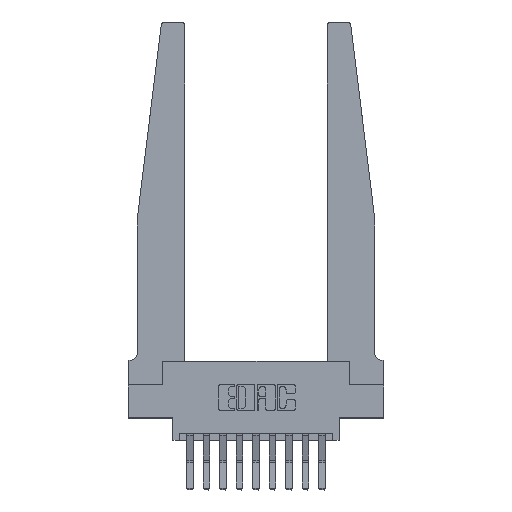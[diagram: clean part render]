
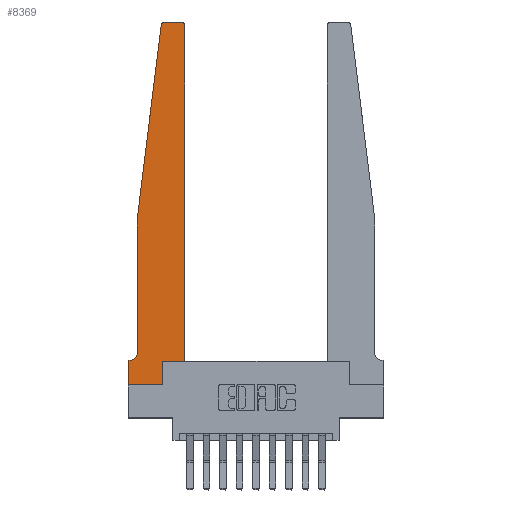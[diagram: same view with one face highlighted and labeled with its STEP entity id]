
A CAD part, top view. The second image highlights one B-rep face of the part: STEP entity #8369.
In plain terms, the highlighted planar face has unit normal (0, 0, 1).
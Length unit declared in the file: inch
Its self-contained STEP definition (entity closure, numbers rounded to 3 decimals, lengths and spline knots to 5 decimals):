
#51 = ORIENTED_EDGE ( 'NONE', *, *, #7504, .T. ) ;
#128 = CARTESIAN_POINT ( 'NONE',  ( 0.425, 0.18, 0.37 ) ) ;
#229 = AXIS2_PLACEMENT_3D ( 'NONE', #2099, #6623, #13943 ) ;
#252 = AXIS2_PLACEMENT_3D ( 'NONE', #6421, #1732, #11304 ) ;
#266 = CARTESIAN_POINT ( 'NONE',  ( 0.065, 1.25, 0.37 ) ) ;
#479 = LINE ( 'NONE', #1680, #1055 ) ;
#628 = AXIS2_PLACEMENT_3D ( 'NONE', #4813, #907, #8316 ) ;
#907 = DIRECTION ( 'NONE',  ( 0., 0., -1. ) ) ;
#963 = ORIENTED_EDGE ( 'NONE', *, *, #7296, .T. ) ;
#1006 = VECTOR ( 'NONE', #1713, 39.37008 ) ;
#1055 = VECTOR ( 'NONE', #5318, 39.37008 ) ;
#1065 = DIRECTION ( 'NONE',  ( -0.122, -0.992, 0. ) ) ;
#1325 = CARTESIAN_POINT ( 'NONE',  ( 0.2605, 0., 0.37 ) ) ;
#1422 = EDGE_CURVE ( 'NONE', #2027, #12959, #5453, .T. ) ;
#1680 = CARTESIAN_POINT ( 'NONE',  ( 0.065, 0.1875, 0.37 ) ) ;
#1713 = DIRECTION ( 'NONE',  ( 0., 1., 0. ) ) ;
#1732 = DIRECTION ( 'NONE',  ( 0., 0., 1. ) ) ;
#1823 = CARTESIAN_POINT ( 'NONE',  ( 0., 0., 0.37 ) ) ;
#1824 = EDGE_CURVE ( 'NONE', #10791, #3498, #9558, .T. ) ;
#2027 = VERTEX_POINT ( 'NONE', #6662 ) ;
#2099 = CARTESIAN_POINT ( 'NONE',  ( 0.27653, 2.72, 0.37 ) ) ;
#2105 = VERTEX_POINT ( 'NONE', #4064 ) ;
#2172 = LINE ( 'NONE', #5431, #9695 ) ;
#2259 = DIRECTION ( 'NONE',  ( 0., 0., 1. ) ) ;
#2354 = LINE ( 'NONE', #9746, #4306 ) ;
#2360 = VERTEX_POINT ( 'NONE', #2491 ) ;
#2491 = CARTESIAN_POINT ( 'NONE',  ( 0.27653, 2.75, 0.37 ) ) ;
#2836 = LINE ( 'NONE', #128, #1006 ) ;
#3005 = EDGE_CURVE ( 'NONE', #14309, #2027, #2172, .T. ) ;
#3423 = EDGE_CURVE ( 'NONE', #12959, #12888, #479, .T. ) ;
#3498 = VERTEX_POINT ( 'NONE', #15337 ) ;
#3895 = VERTEX_POINT ( 'NONE', #13203 ) ;
#4064 = CARTESIAN_POINT ( 'NONE',  ( 0., 0., 0.37 ) ) ;
#4283 = CIRCLE ( 'NONE', #229, 0.03 ) ;
#4306 = VECTOR ( 'NONE', #1065, 39.37008 ) ;
#4813 = CARTESIAN_POINT ( 'NONE',  ( 0.015, 0.2375, 0.37 ) ) ;
#5318 = DIRECTION ( 'NONE',  ( -1., 0., 0. ) ) ;
#5431 = CARTESIAN_POINT ( 'NONE',  ( 0.065, 1.25, 0.37 ) ) ;
#5453 = CIRCLE ( 'NONE', #628, 0.05 ) ;
#5802 = CARTESIAN_POINT ( 'NONE',  ( 0.2605, 0.18, 0.37 ) ) ;
#5808 = CARTESIAN_POINT ( 'NONE',  ( 0., 0.1875, 0.37 ) ) ;
#5860 = DIRECTION ( 'NONE',  ( -1., 0., 0. ) ) ;
#6004 = DIRECTION ( 'NONE',  ( 1., 0., 0. ) ) ;
#6421 = CARTESIAN_POINT ( 'NONE',  ( 0.395, 2.72, 0.37 ) ) ;
#6623 = DIRECTION ( 'NONE',  ( 0., 0., 1. ) ) ;
#6662 = CARTESIAN_POINT ( 'NONE',  ( 0.065, 0.2375, 0.37 ) ) ;
#6698 = VECTOR ( 'NONE', #5860, 39.37008 ) ;
#6762 = EDGE_CURVE ( 'NONE', #12888, #2105, #10340, .T. ) ;
#6911 = VERTEX_POINT ( 'NONE', #7382 ) ;
#7009 = FACE_OUTER_BOUND ( 'NONE', #15376, .T. ) ;
#7210 = LINE ( 'NONE', #9767, #8859 ) ;
#7296 = EDGE_CURVE ( 'NONE', #2105, #10791, #7210, .T. ) ;
#7382 = CARTESIAN_POINT ( 'NONE',  ( 0.425, 2.72, 0.37 ) ) ;
#7504 = EDGE_CURVE ( 'NONE', #8425, #6911, #2836, .T. ) ;
#7798 = EDGE_CURVE ( 'NONE', #3895, #14309, #2354, .T. ) ;
#7845 = VECTOR ( 'NONE', #15487, 39.37008 ) ;
#8140 = CARTESIAN_POINT ( 'NONE',  ( 0., 0.1875, 0.37 ) ) ;
#8253 = ORIENTED_EDGE ( 'NONE', *, *, #3423, .T. ) ;
#8300 = DIRECTION ( 'NONE',  ( 1., 0., 0. ) ) ;
#8316 = DIRECTION ( 'NONE',  ( -1., 0., 0. ) ) ;
#8369 = ADVANCED_FACE ( 'NONE', ( #7009 ), #11893, .T. ) ;
#8425 = VERTEX_POINT ( 'NONE', #12142 ) ;
#8859 = VECTOR ( 'NONE', #6004, 39.37008 ) ;
#9244 = ORIENTED_EDGE ( 'NONE', *, *, #11527, .T. ) ;
#9558 = LINE ( 'NONE', #5802, #10575 ) ;
#9648 = VERTEX_POINT ( 'NONE', #14576 ) ;
#9649 = CIRCLE ( 'NONE', #252, 0.03 ) ;
#9695 = VECTOR ( 'NONE', #14242, 39.37008 ) ;
#9746 = CARTESIAN_POINT ( 'NONE',  ( 0.065, 1.25, 0.37 ) ) ;
#9767 = CARTESIAN_POINT ( 'NONE',  ( 0., 0., 0.37 ) ) ;
#9883 = ORIENTED_EDGE ( 'NONE', *, *, #1422, .T. ) ;
#10250 = CARTESIAN_POINT ( 'NONE',  ( 0.425, 0.18, 0.37 ) ) ;
#10254 = ORIENTED_EDGE ( 'NONE', *, *, #12353, .T. ) ;
#10340 = LINE ( 'NONE', #1823, #7845 ) ;
#10423 = AXIS2_PLACEMENT_3D ( 'NONE', #5808, #2259, #8300 ) ;
#10575 = VECTOR ( 'NONE', #10870, 39.37008 ) ;
#10581 = ORIENTED_EDGE ( 'NONE', *, *, #7798, .T. ) ;
#10791 = VERTEX_POINT ( 'NONE', #1325 ) ;
#10854 = ORIENTED_EDGE ( 'NONE', *, *, #6762, .T. ) ;
#10861 = ORIENTED_EDGE ( 'NONE', *, *, #13412, .T. ) ;
#10870 = DIRECTION ( 'NONE',  ( 0., 1., 0. ) ) ;
#10994 = ORIENTED_EDGE ( 'NONE', *, *, #12763, .T. ) ;
#11128 = ORIENTED_EDGE ( 'NONE', *, *, #3005, .T. ) ;
#11304 = DIRECTION ( 'NONE',  ( 1., 0., 0. ) ) ;
#11527 = EDGE_CURVE ( 'NONE', #9648, #2360, #13042, .T. ) ;
#11893 = PLANE ( 'NONE',  #10423 ) ;
#12142 = CARTESIAN_POINT ( 'NONE',  ( 0.425, 0.18, 0.37 ) ) ;
#12256 = VECTOR ( 'NONE', #15086, 39.37008 ) ;
#12353 = EDGE_CURVE ( 'NONE', #3498, #8425, #13819, .T. ) ;
#12763 = EDGE_CURVE ( 'NONE', #2360, #3895, #4283, .T. ) ;
#12888 = VERTEX_POINT ( 'NONE', #8140 ) ;
#12959 = VERTEX_POINT ( 'NONE', #15623 ) ;
#13042 = LINE ( 'NONE', #15485, #6698 ) ;
#13203 = CARTESIAN_POINT ( 'NONE',  ( 0.24675, 2.72367, 0.37 ) ) ;
#13412 = EDGE_CURVE ( 'NONE', #6911, #9648, #9649, .T. ) ;
#13819 = LINE ( 'NONE', #10250, #12256 ) ;
#13943 = DIRECTION ( 'NONE',  ( 1., 0., 0. ) ) ;
#14242 = DIRECTION ( 'NONE',  ( 0., -1., 0. ) ) ;
#14309 = VERTEX_POINT ( 'NONE', #266 ) ;
#14576 = CARTESIAN_POINT ( 'NONE',  ( 0.395, 2.75, 0.37 ) ) ;
#15086 = DIRECTION ( 'NONE',  ( 1., 0., 0. ) ) ;
#15322 = ORIENTED_EDGE ( 'NONE', *, *, #1824, .T. ) ;
#15337 = CARTESIAN_POINT ( 'NONE',  ( 0.2605, 0.18, 0.37 ) ) ;
#15376 = EDGE_LOOP ( 'NONE', ( #9244, #10994, #10581, #11128, #9883, #8253, #10854, #963, #15322, #10254, #51, #10861 ) ) ;
#15485 = CARTESIAN_POINT ( 'NONE',  ( 0.25, 2.75, 0.37 ) ) ;
#15487 = DIRECTION ( 'NONE',  ( 0., -1., 0. ) ) ;
#15623 = CARTESIAN_POINT ( 'NONE',  ( 0.015, 0.1875, 0.37 ) ) ;
